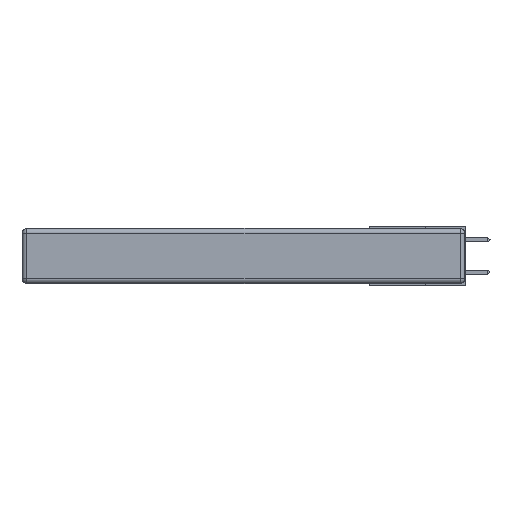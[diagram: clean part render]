
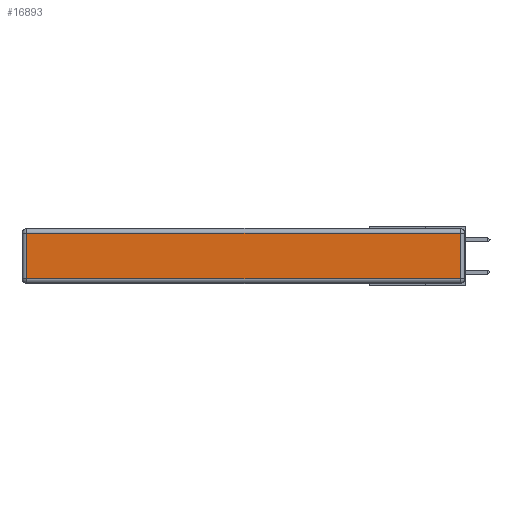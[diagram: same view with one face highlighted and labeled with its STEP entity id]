
A CAD part, left-side view. The second image highlights one B-rep face of the part: STEP entity #16893.
In plain terms, the highlighted planar face has unit normal (-1, 0, 0).
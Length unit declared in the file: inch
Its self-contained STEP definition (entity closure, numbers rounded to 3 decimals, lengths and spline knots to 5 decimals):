
#227 = LINE ( 'NONE', #8030, #10530 ) ;
#350 = VERTEX_POINT ( 'NONE', #10796 ) ;
#778 = FACE_OUTER_BOUND ( 'NONE', #10558, .T. ) ;
#1466 = ORIENTED_EDGE ( 'NONE', *, *, #5469, .T. ) ;
#1547 = EDGE_CURVE ( 'NONE', #21802, #9220, #21246, .T. ) ;
#1982 = EDGE_CURVE ( 'NONE', #350, #21802, #15309, .T. ) ;
#3000 = DIRECTION ( 'NONE',  ( 0., 0., -1. ) ) ;
#3271 = EDGE_CURVE ( 'NONE', #9220, #8665, #18230, .T. ) ;
#3990 = CARTESIAN_POINT ( 'NONE',  ( 0., 0.03, -0.343 ) ) ;
#4395 = DIRECTION ( 'NONE',  ( 0., -1., 0. ) ) ;
#4678 = AXIS2_PLACEMENT_3D ( 'NONE', #16086, #5475, #10565 ) ;
#5469 = EDGE_CURVE ( 'NONE', #8665, #350, #227, .T. ) ;
#5475 = DIRECTION ( 'NONE',  ( -1., 0., 0. ) ) ;
#5792 = ORIENTED_EDGE ( 'NONE', *, *, #3271, .T. ) ;
#6019 = CARTESIAN_POINT ( 'NONE',  ( 0., 0.03, -0.03 ) ) ;
#7677 = CARTESIAN_POINT ( 'NONE',  ( 0., 0., -0.313 ) ) ;
#7982 = DIRECTION ( 'NONE',  ( 0., 1., 0. ) ) ;
#8030 = CARTESIAN_POINT ( 'NONE',  ( 0., 2.72, -0.343 ) ) ;
#8273 = VECTOR ( 'NONE', #4395, 39.37008 ) ;
#8665 = VERTEX_POINT ( 'NONE', #16442 ) ;
#9220 = VERTEX_POINT ( 'NONE', #6019 ) ;
#10530 = VECTOR ( 'NONE', #3000, 39.37008 ) ;
#10558 = EDGE_LOOP ( 'NONE', ( #16928, #21344, #5792, #1466 ) ) ;
#10565 = DIRECTION ( 'NONE',  ( 0., 0., 1. ) ) ;
#10796 = CARTESIAN_POINT ( 'NONE',  ( 0., 2.72, -0.313 ) ) ;
#14355 = DIRECTION ( 'NONE',  ( 0., 0., 1. ) ) ;
#15309 = LINE ( 'NONE', #7677, #8273 ) ;
#16086 = CARTESIAN_POINT ( 'NONE',  ( 0., 0., -0.343 ) ) ;
#16442 = CARTESIAN_POINT ( 'NONE',  ( 0., 2.72, -0.03 ) ) ;
#16529 = CARTESIAN_POINT ( 'NONE',  ( 0., 2.75, -0.03 ) ) ;
#16893 = ADVANCED_FACE ( 'NONE', ( #778 ), #21022, .T. ) ;
#16928 = ORIENTED_EDGE ( 'NONE', *, *, #1982, .T. ) ;
#18230 = LINE ( 'NONE', #16529, #20146 ) ;
#19052 = CARTESIAN_POINT ( 'NONE',  ( 0., 0.03, -0.313 ) ) ;
#20146 = VECTOR ( 'NONE', #7982, 39.37008 ) ;
#21022 = PLANE ( 'NONE',  #4678 ) ;
#21246 = LINE ( 'NONE', #3990, #22371 ) ;
#21344 = ORIENTED_EDGE ( 'NONE', *, *, #1547, .T. ) ;
#21802 = VERTEX_POINT ( 'NONE', #19052 ) ;
#22371 = VECTOR ( 'NONE', #14355, 39.37008 ) ;
